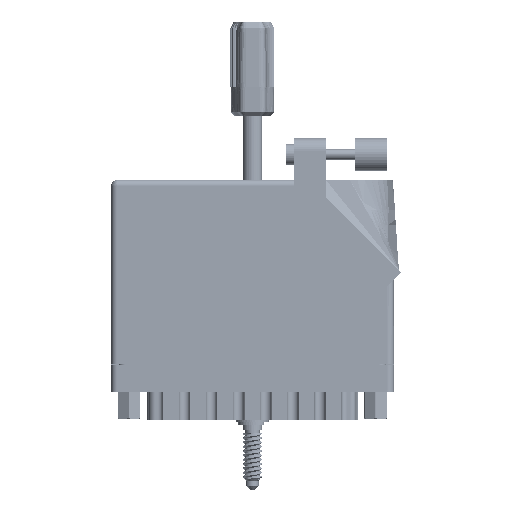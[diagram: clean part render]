
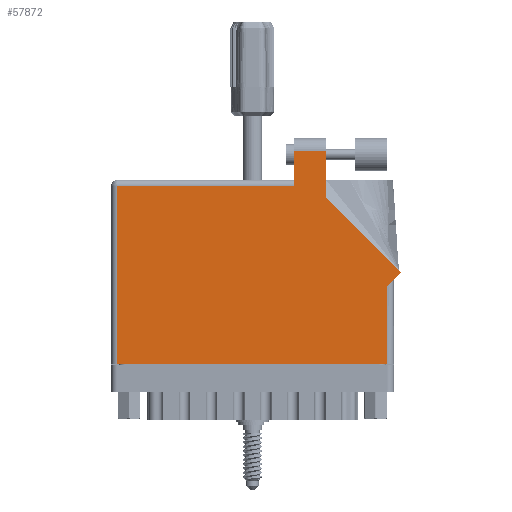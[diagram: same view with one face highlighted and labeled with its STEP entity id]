
A CAD part, front view. The second image highlights one B-rep face of the part: STEP entity #57872.
In plain terms, the highlighted face is planar.
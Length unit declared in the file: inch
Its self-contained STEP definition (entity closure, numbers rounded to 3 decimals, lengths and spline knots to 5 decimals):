
#1009 = CARTESIAN_POINT ( 'NONE',  ( 0., 1.713, 0. ) ) ;
#2676 = VECTOR ( 'NONE', #41182, 39.37008 ) ;
#4300 = CARTESIAN_POINT ( 'NONE',  ( 1.758, 2.05, 0. ) ) ;
#4686 = EDGE_CURVE ( 'NONE', #5172, #60026, #63069, .T. ) ;
#4866 = CARTESIAN_POINT ( 'NONE',  ( 2.656, 0.815, 0. ) ) ;
#5172 = VERTEX_POINT ( 'NONE', #74680 ) ;
#7036 = VECTOR ( 'NONE', #8030, 39.37008 ) ;
#7883 = DIRECTION ( 'NONE',  ( -1., 0., 0. ) ) ;
#8030 = DIRECTION ( 'NONE',  ( -1., 0., 0. ) ) ;
#8471 = DIRECTION ( 'NONE',  ( 1., 0., 0. ) ) ;
#10822 = LINE ( 'NONE', #81515, #33565 ) ;
#11126 = CARTESIAN_POINT ( 'NONE',  ( 0.062, 1.713, 0. ) ) ;
#11393 = CARTESIAN_POINT ( 'NONE',  ( 2.718, 0.815, 0. ) ) ;
#12154 = CARTESIAN_POINT ( 'NONE',  ( 2.78871, 0.88571, 0. ) ) ;
#12312 = ORIENTED_EDGE ( 'NONE', *, *, #83096, .T. ) ;
#12418 = EDGE_CURVE ( 'NONE', #69397, #5172, #68122, .T. ) ;
#13185 = DIRECTION ( 'NONE',  ( 0., 1., 0. ) ) ;
#14582 = EDGE_CURVE ( 'NONE', #90649, #55889, #66535, .T. ) ;
#14620 = CARTESIAN_POINT ( 'NONE',  ( 0., 1.775, 0. ) ) ;
#14786 = VECTOR ( 'NONE', #13185, 39.37008 ) ;
#14995 = AXIS2_PLACEMENT_3D ( 'NONE', #14620, #45923, #7883 ) ;
#16027 = VECTOR ( 'NONE', #8471, 39.37008 ) ;
#18164 = CARTESIAN_POINT ( 'NONE',  ( 1.758, 2.05, 0. ) ) ;
#18230 = EDGE_LOOP ( 'NONE', ( #76188, #36759, #24091, #68143, #51087, #92365, #25676, #24890, #12312 ) ) ;
#18441 = LINE ( 'NONE', #45512, #16027 ) ;
#19141 = EDGE_CURVE ( 'NONE', #50768, #90649, #81668, .T. ) ;
#19566 = EDGE_CURVE ( 'NONE', #76585, #69397, #82819, .T. ) ;
#21049 = VECTOR ( 'NONE', #24605, 39.37008 ) ;
#21185 = VECTOR ( 'NONE', #87898, 39.37008 ) ;
#24091 = ORIENTED_EDGE ( 'NONE', *, *, #12418, .T. ) ;
#24605 = DIRECTION ( 'NONE',  ( -0.707, 0.707, 0. ) ) ;
#24890 = ORIENTED_EDGE ( 'NONE', *, *, #14582, .T. ) ;
#25676 = ORIENTED_EDGE ( 'NONE', *, *, #19141, .T. ) ;
#29949 = CARTESIAN_POINT ( 'NONE',  ( 0.062, 0., 0. ) ) ;
#33565 = VECTOR ( 'NONE', #97866, 39.37008 ) ;
#33589 = EDGE_CURVE ( 'NONE', #60026, #66755, #10822, .T. ) ;
#36759 = ORIENTED_EDGE ( 'NONE', *, *, #19566, .T. ) ;
#40519 = FACE_OUTER_BOUND ( 'NONE', #18230, .T. ) ;
#41182 = DIRECTION ( 'NONE',  ( -1., 0., 0. ) ) ;
#44041 = LINE ( 'NONE', #74415, #65495 ) ;
#45512 = CARTESIAN_POINT ( 'NONE',  ( 0., 0., 0. ) ) ;
#45923 = DIRECTION ( 'NONE',  ( 0., 0., -1. ) ) ;
#50768 = VERTEX_POINT ( 'NONE', #97335 ) ;
#51087 = ORIENTED_EDGE ( 'NONE', *, *, #33589, .T. ) ;
#55889 = VERTEX_POINT ( 'NONE', #12154 ) ;
#57368 = VECTOR ( 'NONE', #76379, 39.37008 ) ;
#57872 = ADVANCED_FACE ( 'NONE', ( #40519 ), #83414, .F. ) ;
#58986 = EDGE_CURVE ( 'NONE', #89869, #76585, #44041, .T. ) ;
#60026 = VERTEX_POINT ( 'NONE', #11126 ) ;
#63069 = LINE ( 'NONE', #1009, #7036 ) ;
#63862 = CARTESIAN_POINT ( 'NONE',  ( 2.78871, 0.88571, 0. ) ) ;
#65495 = VECTOR ( 'NONE', #67704, 39.37008 ) ;
#66535 = LINE ( 'NONE', #11393, #21185 ) ;
#66755 = VERTEX_POINT ( 'NONE', #29949 ) ;
#67704 = DIRECTION ( 'NONE',  ( 0., 1., 0. ) ) ;
#67938 = EDGE_CURVE ( 'NONE', #66755, #50768, #18441, .T. ) ;
#68122 = LINE ( 'NONE', #84736, #57368 ) ;
#68143 = ORIENTED_EDGE ( 'NONE', *, *, #4686, .T. ) ;
#69397 = VERTEX_POINT ( 'NONE', #4300 ) ;
#72445 = LINE ( 'NONE', #63862, #21049 ) ;
#74415 = CARTESIAN_POINT ( 'NONE',  ( 2.065, 1.60942, 0. ) ) ;
#74680 = CARTESIAN_POINT ( 'NONE',  ( 1.758, 1.713, 0. ) ) ;
#76188 = ORIENTED_EDGE ( 'NONE', *, *, #58986, .T. ) ;
#76379 = DIRECTION ( 'NONE',  ( 0., -1., 0. ) ) ;
#76585 = VERTEX_POINT ( 'NONE', #92673 ) ;
#81515 = CARTESIAN_POINT ( 'NONE',  ( 0.062, 0., 0. ) ) ;
#81668 = LINE ( 'NONE', #4866, #14786 ) ;
#82819 = LINE ( 'NONE', #18164, #2676 ) ;
#83096 = EDGE_CURVE ( 'NONE', #55889, #89869, #72445, .T. ) ;
#83414 = PLANE ( 'NONE',  #14995 ) ;
#84736 = CARTESIAN_POINT ( 'NONE',  ( 1.758, 1.775, 0. ) ) ;
#87898 = DIRECTION ( 'NONE',  ( 0.707, 0.707, 0. ) ) ;
#89869 = VERTEX_POINT ( 'NONE', #94399 ) ;
#90649 = VERTEX_POINT ( 'NONE', #90929 ) ;
#90929 = CARTESIAN_POINT ( 'NONE',  ( 2.656, 0.753, 0. ) ) ;
#92365 = ORIENTED_EDGE ( 'NONE', *, *, #67938, .T. ) ;
#92673 = CARTESIAN_POINT ( 'NONE',  ( 2.065, 2.05, 0. ) ) ;
#94399 = CARTESIAN_POINT ( 'NONE',  ( 2.065, 1.60942, 0. ) ) ;
#97335 = CARTESIAN_POINT ( 'NONE',  ( 2.656, 0., 0. ) ) ;
#97866 = DIRECTION ( 'NONE',  ( 0., -1., 0. ) ) ;
